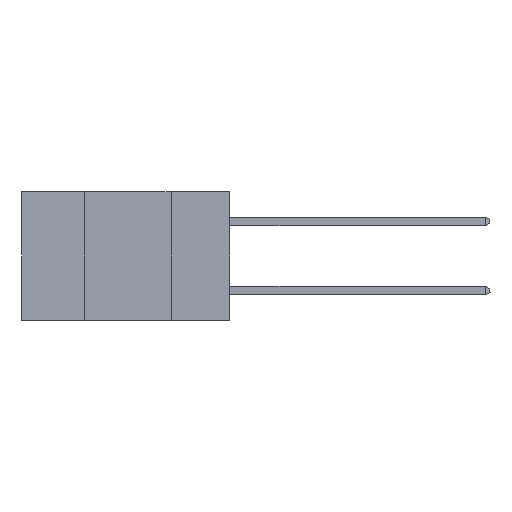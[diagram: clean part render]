
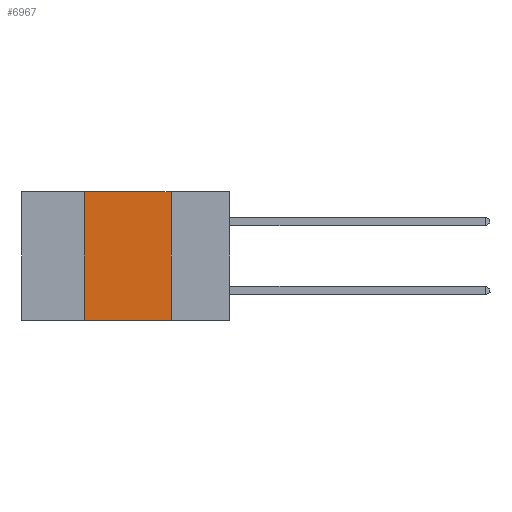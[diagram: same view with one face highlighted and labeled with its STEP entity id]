
A CAD part, left-side view. The second image highlights one B-rep face of the part: STEP entity #6967.
In plain terms, the highlighted planar face has unit normal (-1, 0, 0).
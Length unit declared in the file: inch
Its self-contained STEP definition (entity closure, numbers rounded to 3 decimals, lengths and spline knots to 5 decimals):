
#312 = CARTESIAN_POINT ( 'NONE',  ( 0., 0.17, 0. ) ) ;
#799 = VERTEX_POINT ( 'NONE', #8852 ) ;
#802 = VERTEX_POINT ( 'NONE', #8661 ) ;
#1016 = CARTESIAN_POINT ( 'NONE',  ( 0., 0.6, 0. ) ) ;
#1094 = EDGE_CURVE ( 'NONE', #802, #5117, #3028, .T. ) ;
#1305 = ORIENTED_EDGE ( 'NONE', *, *, #1094, .F. ) ;
#1998 = DIRECTION ( 'NONE',  ( 0., -1., 0. ) ) ;
#2293 = AXIS2_PLACEMENT_3D ( 'NONE', #5470, #5366, #8980 ) ;
#2828 = PLANE ( 'NONE',  #2293 ) ;
#2871 = DIRECTION ( 'NONE',  ( 0., -1., 0. ) ) ;
#3028 = LINE ( 'NONE', #13762, #6150 ) ;
#3213 = LINE ( 'NONE', #9444, #12177 ) ;
#4234 = LINE ( 'NONE', #9904, #13357 ) ;
#5117 = VERTEX_POINT ( 'NONE', #12689 ) ;
#5366 = DIRECTION ( 'NONE',  ( 1., 0., 0. ) ) ;
#5470 = CARTESIAN_POINT ( 'NONE',  ( 0., 0.6, 0. ) ) ;
#5865 = EDGE_LOOP ( 'NONE', ( #6558, #10778, #1305, #9759 ) ) ;
#6048 = VECTOR ( 'NONE', #1998, 39.37008 ) ;
#6150 = VECTOR ( 'NONE', #6798, 39.37008 ) ;
#6462 = VERTEX_POINT ( 'NONE', #312 ) ;
#6558 = ORIENTED_EDGE ( 'NONE', *, *, #6769, .F. ) ;
#6769 = EDGE_CURVE ( 'NONE', #6462, #799, #3213, .T. ) ;
#6798 = DIRECTION ( 'NONE',  ( 0., 0., 1. ) ) ;
#6967 = ADVANCED_FACE ( 'NONE', ( #11433 ), #2828, .F. ) ;
#8661 = CARTESIAN_POINT ( 'NONE',  ( 0., 0.42, -0.37 ) ) ;
#8852 = CARTESIAN_POINT ( 'NONE',  ( 0., 0.17, -0.37 ) ) ;
#8953 = EDGE_CURVE ( 'NONE', #802, #799, #4234, .T. ) ;
#8980 = DIRECTION ( 'NONE',  ( 0., 0., -1. ) ) ;
#9157 = LINE ( 'NONE', #1016, #6048 ) ;
#9244 = EDGE_CURVE ( 'NONE', #5117, #6462, #9157, .T. ) ;
#9444 = CARTESIAN_POINT ( 'NONE',  ( 0., 0.17, 0. ) ) ;
#9759 = ORIENTED_EDGE ( 'NONE', *, *, #8953, .T. ) ;
#9904 = CARTESIAN_POINT ( 'NONE',  ( 0., 0.6, -0.37 ) ) ;
#10778 = ORIENTED_EDGE ( 'NONE', *, *, #9244, .F. ) ;
#11433 = FACE_OUTER_BOUND ( 'NONE', #5865, .T. ) ;
#11644 = DIRECTION ( 'NONE',  ( 0., 0., -1. ) ) ;
#12177 = VECTOR ( 'NONE', #11644, 39.37008 ) ;
#12689 = CARTESIAN_POINT ( 'NONE',  ( 0., 0.42, 0. ) ) ;
#13357 = VECTOR ( 'NONE', #2871, 39.37008 ) ;
#13762 = CARTESIAN_POINT ( 'NONE',  ( 0., 0.42, 0. ) ) ;
